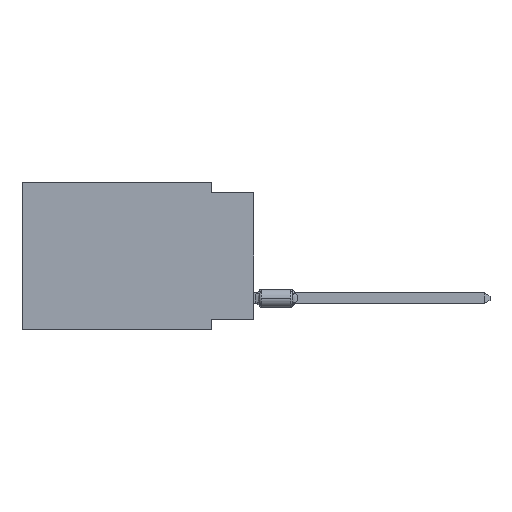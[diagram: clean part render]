
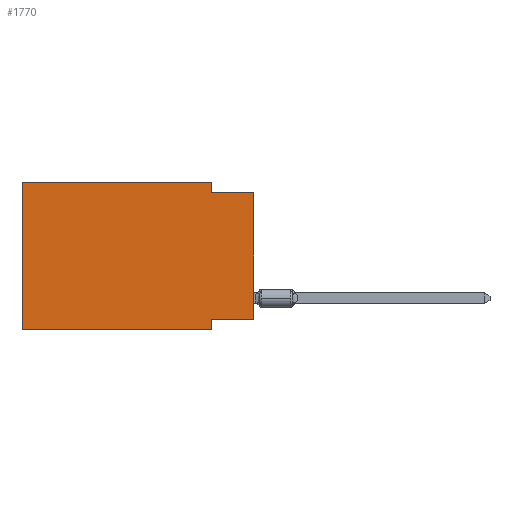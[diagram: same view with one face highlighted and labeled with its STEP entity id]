
A CAD part, left-side view. The second image highlights one B-rep face of the part: STEP entity #1770.
In plain terms, the highlighted planar face has unit normal (-1, 0, 0).
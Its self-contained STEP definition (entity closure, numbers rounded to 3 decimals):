
#118 = ORIENTED_EDGE ( 'NONE', *, *, #10630, .F. ) ;
#460 = CARTESIAN_POINT ( 'NONE',  ( 0., 2.54, 0. ) ) ;
#1770 = ADVANCED_FACE ( 'NONE', ( #2420 ), #13854, .F. ) ;
#2400 = DIRECTION ( 'NONE',  ( 0., 1., 0. ) ) ;
#2420 = FACE_OUTER_BOUND ( 'NONE', #5791, .T. ) ;
#2571 = ORIENTED_EDGE ( 'NONE', *, *, #7375, .F. ) ;
#2647 = VERTEX_POINT ( 'NONE', #6477 ) ;
#2881 = CARTESIAN_POINT ( 'NONE',  ( 0., 13.97, -8.89 ) ) ;
#3676 = ORIENTED_EDGE ( 'NONE', *, *, #17751, .F. ) ;
#3686 = CARTESIAN_POINT ( 'NONE',  ( 0., 13.97, -8.89 ) ) ;
#4085 = DIRECTION ( 'NONE',  ( 1., 0., 0. ) ) ;
#4294 = DIRECTION ( 'NONE',  ( 0., 0., 1. ) ) ;
#4978 = ORIENTED_EDGE ( 'NONE', *, *, #13472, .F. ) ;
#5448 = LINE ( 'NONE', #12915, #13190 ) ;
#5491 = CARTESIAN_POINT ( 'NONE',  ( 0., 2.54, -8.255 ) ) ;
#5601 = VECTOR ( 'NONE', #17068, 1000. ) ;
#5698 = ORIENTED_EDGE ( 'NONE', *, *, #10479, .T. ) ;
#5791 = EDGE_LOOP ( 'NONE', ( #14327, #3676, #4978, #10887, #14368, #5698, #2571, #118 ) ) ;
#5804 = CARTESIAN_POINT ( 'NONE',  ( 0., 0., -8.255 ) ) ;
#6477 = CARTESIAN_POINT ( 'NONE',  ( 0., 2.54, -8.89 ) ) ;
#6622 = DIRECTION ( 'NONE',  ( 0., 0., -1. ) ) ;
#7044 = CARTESIAN_POINT ( 'NONE',  ( 0., 13.97, 0. ) ) ;
#7375 = EDGE_CURVE ( 'NONE', #16152, #2647, #18178, .T. ) ;
#7679 = LINE ( 'NONE', #460, #14697 ) ;
#8344 = CARTESIAN_POINT ( 'NONE',  ( 0., 2.54, -0.635 ) ) ;
#9382 = VERTEX_POINT ( 'NONE', #7044 ) ;
#10003 = DIRECTION ( 'NONE',  ( 0., 0., -1. ) ) ;
#10476 = VECTOR ( 'NONE', #20482, 1000. ) ;
#10479 = EDGE_CURVE ( 'NONE', #11234, #2647, #13341, .T. ) ;
#10630 = EDGE_CURVE ( 'NONE', #22493, #16152, #11911, .T. ) ;
#10887 = ORIENTED_EDGE ( 'NONE', *, *, #19398, .F. ) ;
#11234 = VERTEX_POINT ( 'NONE', #2881 ) ;
#11703 = DIRECTION ( 'NONE',  ( 0., -1., 0. ) ) ;
#11815 = LINE ( 'NONE', #15540, #12929 ) ;
#11911 = LINE ( 'NONE', #12169, #12181 ) ;
#12169 = CARTESIAN_POINT ( 'NONE',  ( 0., 0., -8.255 ) ) ;
#12181 = VECTOR ( 'NONE', #2400, 1000. ) ;
#12915 = CARTESIAN_POINT ( 'NONE',  ( 0., 0., -0.635 ) ) ;
#12929 = VECTOR ( 'NONE', #13871, 1000. ) ;
#13073 = VERTEX_POINT ( 'NONE', #14139 ) ;
#13190 = VECTOR ( 'NONE', #16894, 1000. ) ;
#13341 = LINE ( 'NONE', #3686, #5601 ) ;
#13472 = EDGE_CURVE ( 'NONE', #13073, #24441, #7679, .T. ) ;
#13854 = PLANE ( 'NONE',  #18512 ) ;
#13871 = DIRECTION ( 'NONE',  ( 0., 0., 1. ) ) ;
#13979 = CARTESIAN_POINT ( 'NONE',  ( 0., 13.97, 0. ) ) ;
#14139 = CARTESIAN_POINT ( 'NONE',  ( 0., 2.54, 0. ) ) ;
#14327 = ORIENTED_EDGE ( 'NONE', *, *, #23384, .T. ) ;
#14368 = ORIENTED_EDGE ( 'NONE', *, *, #24256, .F. ) ;
#14697 = VECTOR ( 'NONE', #6622, 1000. ) ;
#15476 = LINE ( 'NONE', #15984, #21115 ) ;
#15540 = CARTESIAN_POINT ( 'NONE',  ( 0., 13.97, 0. ) ) ;
#15984 = CARTESIAN_POINT ( 'NONE',  ( 0., 0., 0. ) ) ;
#16152 = VERTEX_POINT ( 'NONE', #5491 ) ;
#16894 = DIRECTION ( 'NONE',  ( 0., -1., 0. ) ) ;
#17068 = DIRECTION ( 'NONE',  ( 0., -1., 0. ) ) ;
#17751 = EDGE_CURVE ( 'NONE', #24441, #19680, #5448, .T. ) ;
#18178 = LINE ( 'NONE', #24473, #10476 ) ;
#18512 = AXIS2_PLACEMENT_3D ( 'NONE', #13979, #4085, #10003 ) ;
#19398 = EDGE_CURVE ( 'NONE', #9382, #13073, #25320, .T. ) ;
#19680 = VERTEX_POINT ( 'NONE', #24931 ) ;
#20482 = DIRECTION ( 'NONE',  ( 0., 0., -1. ) ) ;
#21115 = VECTOR ( 'NONE', #4294, 1000. ) ;
#21462 = CARTESIAN_POINT ( 'NONE',  ( 0., 13.97, 0. ) ) ;
#22493 = VERTEX_POINT ( 'NONE', #5804 ) ;
#23384 = EDGE_CURVE ( 'NONE', #22493, #19680, #15476, .T. ) ;
#23873 = VECTOR ( 'NONE', #11703, 1000. ) ;
#24256 = EDGE_CURVE ( 'NONE', #11234, #9382, #11815, .T. ) ;
#24441 = VERTEX_POINT ( 'NONE', #8344 ) ;
#24473 = CARTESIAN_POINT ( 'NONE',  ( 0., 2.54, -8.89 ) ) ;
#24931 = CARTESIAN_POINT ( 'NONE',  ( 0., 0., -0.635 ) ) ;
#25320 = LINE ( 'NONE', #21462, #23873 ) ;
